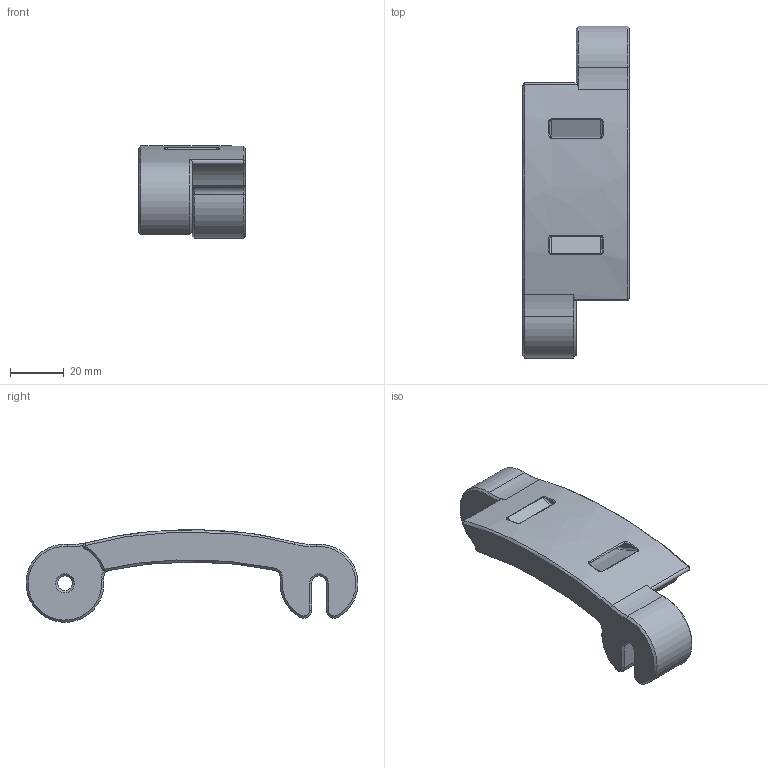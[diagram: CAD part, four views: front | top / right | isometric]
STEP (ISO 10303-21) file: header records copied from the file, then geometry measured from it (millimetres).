
FILE_DESCRIPTION (( 'STEP AP203' ), '1' );
FILE_NAME ('WTF-9_stock_brace_1.STEP', '2020-05-09T10:20:35', ( '' ), ( '' ), 'SwSTEP 2.0', 'SolidWorks 2016', '' );
FILE_SCHEMA (( 'CONFIG_CONTROL_DESIGN' ));
Length unit declared in the file: millimetre
Products named in the file (2): WTF9 V1 FINAL_18; WTF-9_stock_brace_1
Assembly tree (1 placements, depth 2):
  WTF-9_stock_brace_1
    WTF9 V1 FINAL_18
Bounding box: 40 x 124.12 x 34.55 mm (x, y, z)
Volume: 57110.7 mm3; surface area: 16171.7 mm2
Topology: 1 solids, 1 shells, 85 faces, 199 edges, 116 vertices
Faces by surface type: bspline 31, cone 23, cylinder 15, plane 12, torus 4
Full cylindrical faces by diameter (mm): 5.5 x1
Entity records: 3636 total; most frequent: CARTESIAN_POINT 1711, ORIENTED_EDGE 392, DIRECTION 300, EDGE_CURVE 196, AXIS2_PLACEMENT_3D 116, VERTEX_POINT 116, EDGE_LOOP 92, FACE_OUTER_BOUND 86
